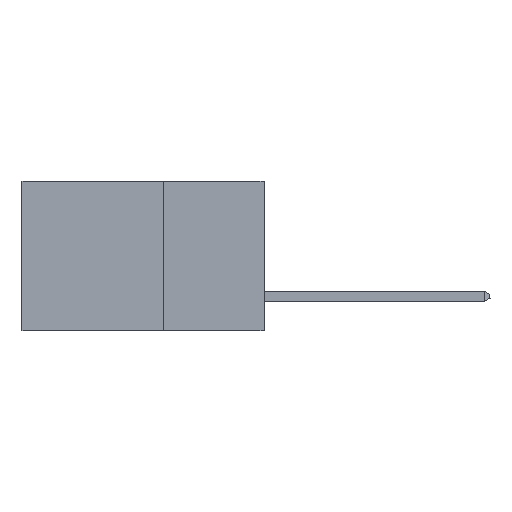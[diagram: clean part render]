
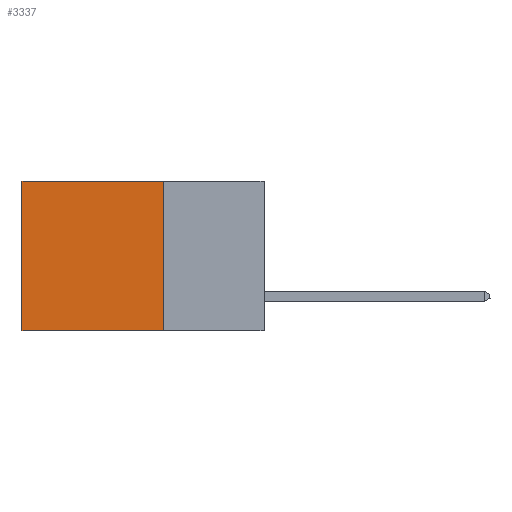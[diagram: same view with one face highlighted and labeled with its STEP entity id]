
A CAD part, left-side view. The second image highlights one B-rep face of the part: STEP entity #3337.
In plain terms, the highlighted planar face has unit normal (-1, 0, 0).
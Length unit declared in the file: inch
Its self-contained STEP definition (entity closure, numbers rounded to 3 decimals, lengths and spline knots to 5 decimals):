
#586 = DIRECTION ( 'NONE',  ( 0., 0., -1. ) ) ;
#728 = EDGE_CURVE ( 'NONE', #7013, #2680, #3792, .T. ) ;
#781 = CARTESIAN_POINT ( 'NONE',  ( 0.298, 0.25, -0.37 ) ) ;
#1291 = EDGE_LOOP ( 'NONE', ( #8799, #8978, #8888, #8941 ) ) ;
#1378 = FACE_OUTER_BOUND ( 'NONE', #1291, .T. ) ;
#1415 = CARTESIAN_POINT ( 'NONE',  ( 0.298, 0.25, 0. ) ) ;
#1597 = CARTESIAN_POINT ( 'NONE',  ( 0.298, 0.25, 0. ) ) ;
#1719 = CARTESIAN_POINT ( 'NONE',  ( 0.298, 0.25, 0. ) ) ;
#1739 = CARTESIAN_POINT ( 'NONE',  ( 0.298, 0.25, 0. ) ) ;
#2028 = EDGE_CURVE ( 'NONE', #5334, #7013, #3952, .T. ) ;
#2621 = VECTOR ( 'NONE', #8420, 39.37008 ) ;
#2680 = VERTEX_POINT ( 'NONE', #6233 ) ;
#3337 = ADVANCED_FACE ( 'NONE', ( #1378 ), #4170, .F. ) ;
#3792 = LINE ( 'NONE', #781, #7330 ) ;
#3952 = LINE ( 'NONE', #1597, #5615 ) ;
#4053 = DIRECTION ( 'NONE',  ( 0., 0., -1. ) ) ;
#4170 = PLANE ( 'NONE',  #4824 ) ;
#4285 = DIRECTION ( 'NONE',  ( 1., 0., 0. ) ) ;
#4824 = AXIS2_PLACEMENT_3D ( 'NONE', #1415, #4285, #4053 ) ;
#5334 = VERTEX_POINT ( 'NONE', #1739 ) ;
#5615 = VECTOR ( 'NONE', #586, 39.37008 ) ;
#5953 = VECTOR ( 'NONE', #6972, 39.37008 ) ;
#6233 = CARTESIAN_POINT ( 'NONE',  ( 0.298, 0.6, -0.37 ) ) ;
#6886 = EDGE_CURVE ( 'NONE', #6907, #2680, #7847, .T. ) ;
#6907 = VERTEX_POINT ( 'NONE', #7690 ) ;
#6972 = DIRECTION ( 'NONE',  ( 0., 0., -1. ) ) ;
#7013 = VERTEX_POINT ( 'NONE', #7039 ) ;
#7039 = CARTESIAN_POINT ( 'NONE',  ( 0.298, 0.25, -0.37 ) ) ;
#7330 = VECTOR ( 'NONE', #9320, 39.37008 ) ;
#7690 = CARTESIAN_POINT ( 'NONE',  ( 0.298, 0.6, 0. ) ) ;
#7798 = EDGE_CURVE ( 'NONE', #5334, #6907, #8609, .T. ) ;
#7847 = LINE ( 'NONE', #9677, #5953 ) ;
#8420 = DIRECTION ( 'NONE',  ( 0., 1., 0. ) ) ;
#8609 = LINE ( 'NONE', #1719, #2621 ) ;
#8799 = ORIENTED_EDGE ( 'NONE', *, *, #6886, .T. ) ;
#8888 = ORIENTED_EDGE ( 'NONE', *, *, #2028, .F. ) ;
#8941 = ORIENTED_EDGE ( 'NONE', *, *, #7798, .T. ) ;
#8978 = ORIENTED_EDGE ( 'NONE', *, *, #728, .F. ) ;
#9320 = DIRECTION ( 'NONE',  ( 0., 1., 0. ) ) ;
#9677 = CARTESIAN_POINT ( 'NONE',  ( 0.298, 0.6, 0. ) ) ;
